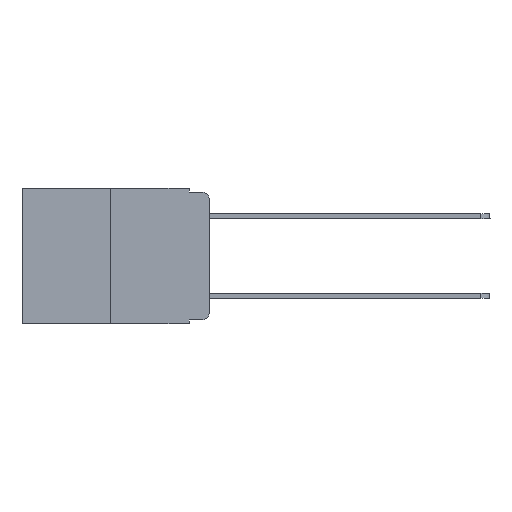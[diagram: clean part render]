
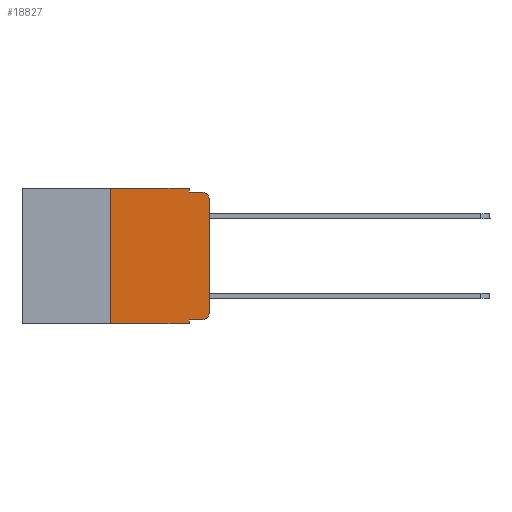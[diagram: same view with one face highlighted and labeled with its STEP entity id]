
A CAD part, left-side view. The second image highlights one B-rep face of the part: STEP entity #18827.
In plain terms, the highlighted planar face has unit normal (-1, 0, 0).
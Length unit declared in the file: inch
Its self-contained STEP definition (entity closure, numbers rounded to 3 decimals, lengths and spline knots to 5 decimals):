
#274 = VERTEX_POINT ( 'NONE', #13769 ) ;
#375 = EDGE_CURVE ( 'NONE', #22445, #3031, #16302, .T. ) ;
#453 = DIRECTION ( 'NONE',  ( 0., 0., -1. ) ) ;
#570 = VECTOR ( 'NONE', #3188, 39.37008 ) ;
#896 = EDGE_CURVE ( 'NONE', #274, #21139, #10821, .T. ) ;
#1306 = LINE ( 'NONE', #13246, #4760 ) ;
#1683 = CARTESIAN_POINT ( 'NONE',  ( 0., 0.473, 0. ) ) ;
#3031 = VERTEX_POINT ( 'NONE', #5684 ) ;
#3120 = CARTESIAN_POINT ( 'NONE',  ( 0., 0.473, -0.343 ) ) ;
#3179 = ORIENTED_EDGE ( 'NONE', *, *, #9342, .T. ) ;
#3188 = DIRECTION ( 'NONE',  ( 0., -1., 0. ) ) ;
#3367 = DIRECTION ( 'NONE',  ( 0., 0., -1. ) ) ;
#3530 = ORIENTED_EDGE ( 'NONE', *, *, #896, .T. ) ;
#4096 = ORIENTED_EDGE ( 'NONE', *, *, #16416, .T. ) ;
#4716 = CARTESIAN_POINT ( 'NONE',  ( 0., 0.02, -0.01 ) ) ;
#4760 = VECTOR ( 'NONE', #18782, 39.37008 ) ;
#5252 = VECTOR ( 'NONE', #3367, 39.37008 ) ;
#5290 = AXIS2_PLACEMENT_3D ( 'NONE', #22202, #11330, #453 ) ;
#5387 = VECTOR ( 'NONE', #15945, 39.37008 ) ;
#5667 = CARTESIAN_POINT ( 'NONE',  ( 0., 0.051, -0.01 ) ) ;
#5684 = CARTESIAN_POINT ( 'NONE',  ( 0., 0.051, -0.343 ) ) ;
#5970 = DIRECTION ( 'NONE',  ( 0., 0., -1. ) ) ;
#6498 = DIRECTION ( 'NONE',  ( 0., 0., 1. ) ) ;
#6510 = CARTESIAN_POINT ( 'NONE',  ( 0., 0.051, 0. ) ) ;
#6875 = CARTESIAN_POINT ( 'NONE',  ( 0., 0.051, -0.333 ) ) ;
#6961 = CARTESIAN_POINT ( 'NONE',  ( 0., 0.051, 0. ) ) ;
#7318 = VERTEX_POINT ( 'NONE', #5667 ) ;
#8241 = CARTESIAN_POINT ( 'NONE',  ( 0., 0.02, -0.333 ) ) ;
#8284 = ORIENTED_EDGE ( 'NONE', *, *, #22790, .F. ) ;
#8750 = FACE_OUTER_BOUND ( 'NONE', #13877, .T. ) ;
#8951 = LINE ( 'NONE', #1683, #11451 ) ;
#9299 = VECTOR ( 'NONE', #6498, 39.37008 ) ;
#9342 = EDGE_CURVE ( 'NONE', #18659, #17824, #11456, .T. ) ;
#9512 = LINE ( 'NONE', #6961, #5252 ) ;
#9538 = CARTESIAN_POINT ( 'NONE',  ( 0., 0.02, -0.313 ) ) ;
#10052 = VERTEX_POINT ( 'NONE', #6510 ) ;
#10553 = VERTEX_POINT ( 'NONE', #22425 ) ;
#10565 = DIRECTION ( 'NONE',  ( 0., 0., -1. ) ) ;
#10660 = ORIENTED_EDGE ( 'NONE', *, *, #12643, .F. ) ;
#10821 = LINE ( 'NONE', #6875, #570 ) ;
#11330 = DIRECTION ( 'NONE',  ( -1., 0., 0. ) ) ;
#11451 = VECTOR ( 'NONE', #21624, 39.37008 ) ;
#11456 = CIRCLE ( 'NONE', #5290, 0.02 ) ;
#11555 = ORIENTED_EDGE ( 'NONE', *, *, #375, .T. ) ;
#12643 = EDGE_CURVE ( 'NONE', #7318, #17824, #19006, .T. ) ;
#13110 = LINE ( 'NONE', #17419, #13687 ) ;
#13246 = CARTESIAN_POINT ( 'NONE',  ( 0., 0.25, 0. ) ) ;
#13687 = VECTOR ( 'NONE', #22970, 39.37008 ) ;
#13769 = CARTESIAN_POINT ( 'NONE',  ( 0., 0.051, -0.333 ) ) ;
#13877 = EDGE_LOOP ( 'NONE', ( #20186, #3179, #10660, #19439, #8284, #21123, #11555, #23515, #3530, #4096 ) ) ;
#14104 = CARTESIAN_POINT ( 'NONE',  ( 0., 0.051, -0.01 ) ) ;
#14159 = DIRECTION ( 'NONE',  ( 0., -1., 0. ) ) ;
#14739 = CARTESIAN_POINT ( 'NONE',  ( 0., 0.25, 0. ) ) ;
#15161 = AXIS2_PLACEMENT_3D ( 'NONE', #17950, #21664, #10565 ) ;
#15834 = LINE ( 'NONE', #19174, #9299 ) ;
#15922 = EDGE_CURVE ( 'NONE', #10052, #7318, #13110, .T. ) ;
#15945 = DIRECTION ( 'NONE',  ( 0., -1., 0. ) ) ;
#16302 = LINE ( 'NONE', #3120, #21647 ) ;
#16416 = EDGE_CURVE ( 'NONE', #21139, #10553, #20989, .T. ) ;
#16838 = DIRECTION ( 'NONE',  ( -1., 0., 0. ) ) ;
#17419 = CARTESIAN_POINT ( 'NONE',  ( 0., 0.051, 0. ) ) ;
#17603 = VERTEX_POINT ( 'NONE', #14739 ) ;
#17824 = VERTEX_POINT ( 'NONE', #4716 ) ;
#17950 = CARTESIAN_POINT ( 'NONE',  ( 0., 0.473, 0. ) ) ;
#18659 = VERTEX_POINT ( 'NONE', #23184 ) ;
#18782 = DIRECTION ( 'NONE',  ( 0., 0., 1. ) ) ;
#18827 = ADVANCED_FACE ( 'NONE', ( #8750 ), #21429, .F. ) ;
#19006 = LINE ( 'NONE', #14104, #5387 ) ;
#19174 = CARTESIAN_POINT ( 'NONE',  ( 0., 0., 0. ) ) ;
#19439 = ORIENTED_EDGE ( 'NONE', *, *, #15922, .F. ) ;
#19987 = EDGE_CURVE ( 'NONE', #274, #3031, #9512, .T. ) ;
#20186 = ORIENTED_EDGE ( 'NONE', *, *, #21104, .T. ) ;
#20539 = AXIS2_PLACEMENT_3D ( 'NONE', #9538, #16838, #5970 ) ;
#20989 = CIRCLE ( 'NONE', #20539, 0.02 ) ;
#21026 = EDGE_CURVE ( 'NONE', #22445, #17603, #1306, .T. ) ;
#21104 = EDGE_CURVE ( 'NONE', #10553, #18659, #15834, .T. ) ;
#21123 = ORIENTED_EDGE ( 'NONE', *, *, #21026, .F. ) ;
#21139 = VERTEX_POINT ( 'NONE', #8241 ) ;
#21429 = PLANE ( 'NONE',  #15161 ) ;
#21624 = DIRECTION ( 'NONE',  ( 0., -1., 0. ) ) ;
#21647 = VECTOR ( 'NONE', #14159, 39.37008 ) ;
#21664 = DIRECTION ( 'NONE',  ( 1., 0., 0. ) ) ;
#22202 = CARTESIAN_POINT ( 'NONE',  ( 0., 0.02, -0.03 ) ) ;
#22425 = CARTESIAN_POINT ( 'NONE',  ( 0., 0., -0.313 ) ) ;
#22445 = VERTEX_POINT ( 'NONE', #22906 ) ;
#22790 = EDGE_CURVE ( 'NONE', #17603, #10052, #8951, .T. ) ;
#22906 = CARTESIAN_POINT ( 'NONE',  ( 0., 0.25, -0.343 ) ) ;
#22970 = DIRECTION ( 'NONE',  ( 0., 0., -1. ) ) ;
#23184 = CARTESIAN_POINT ( 'NONE',  ( 0., 0., -0.03 ) ) ;
#23515 = ORIENTED_EDGE ( 'NONE', *, *, #19987, .F. ) ;
